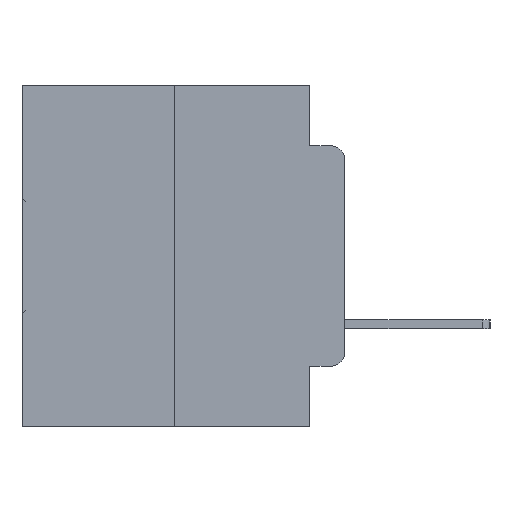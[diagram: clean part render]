
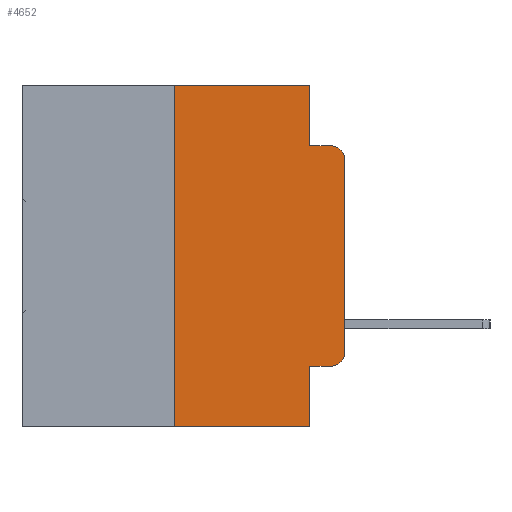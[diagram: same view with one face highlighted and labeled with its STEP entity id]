
A CAD part, left-side view. The second image highlights one B-rep face of the part: STEP entity #4652.
In plain terms, the highlighted planar face has unit normal (-1, 0, 0).
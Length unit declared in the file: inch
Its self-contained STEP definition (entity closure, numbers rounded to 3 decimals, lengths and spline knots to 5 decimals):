
#3 = ORIENTED_EDGE ( 'NONE', *, *, #9504, .F. ) ;
#164 = LINE ( 'NONE', #7670, #29394 ) ;
#460 = EDGE_CURVE ( 'NONE', #24137, #20980, #17345, .T. ) ;
#507 = VERTEX_POINT ( 'NONE', #9055 ) ;
#693 = LINE ( 'NONE', #4307, #24774 ) ;
#829 = VERTEX_POINT ( 'NONE', #10100 ) ;
#1469 = EDGE_CURVE ( 'NONE', #29351, #12513, #18439, .T. ) ;
#1563 = AXIS2_PLACEMENT_3D ( 'NONE', #19869, #17249, #2121 ) ;
#1750 = VECTOR ( 'NONE', #28447, 39.37008 ) ;
#2052 = EDGE_CURVE ( 'NONE', #29351, #24137, #27473, .T. ) ;
#2121 = DIRECTION ( 'NONE',  ( 0., 0., -1. ) ) ;
#2482 = CIRCLE ( 'NONE', #19789, 0.02 ) ;
#4156 = LINE ( 'NONE', #16186, #27305 ) ;
#4307 = CARTESIAN_POINT ( 'NONE',  ( 0., 0.051, -0.0885 ) ) ;
#4398 = LINE ( 'NONE', #22246, #21692 ) ;
#4652 = ADVANCED_FACE ( 'NONE', ( #13198 ), #22043, .F. ) ;
#4811 = ORIENTED_EDGE ( 'NONE', *, *, #11103, .F. ) ;
#5199 = CARTESIAN_POINT ( 'NONE',  ( 0., 0.02, -0.0885 ) ) ;
#5514 = DIRECTION ( 'NONE',  ( 0., 0., -1. ) ) ;
#6791 = DIRECTION ( 'NONE',  ( 0., -1., 0. ) ) ;
#6824 = DIRECTION ( 'NONE',  ( -1., 0., 0. ) ) ;
#7280 = CARTESIAN_POINT ( 'NONE',  ( 0., 0.051, 0. ) ) ;
#7670 = CARTESIAN_POINT ( 'NONE',  ( 0., 0., 0. ) ) ;
#8315 = DIRECTION ( 'NONE',  ( 0., 0., -1. ) ) ;
#8844 = CARTESIAN_POINT ( 'NONE',  ( 0., 0.051, -0.5 ) ) ;
#8852 = CARTESIAN_POINT ( 'NONE',  ( 0., 0.473, 0. ) ) ;
#8989 = ORIENTED_EDGE ( 'NONE', *, *, #18847, .F. ) ;
#8995 = CARTESIAN_POINT ( 'NONE',  ( 0., 0.02, -0.1085 ) ) ;
#9055 = CARTESIAN_POINT ( 'NONE',  ( 0., 0.051, -0.0885 ) ) ;
#9147 = VERTEX_POINT ( 'NONE', #5199 ) ;
#9278 = VECTOR ( 'NONE', #13189, 39.37008 ) ;
#9386 = DIRECTION ( 'NONE',  ( 0., 0., -1. ) ) ;
#9387 = ORIENTED_EDGE ( 'NONE', *, *, #1469, .F. ) ;
#9504 = EDGE_CURVE ( 'NONE', #16824, #829, #4156, .T. ) ;
#10100 = CARTESIAN_POINT ( 'NONE',  ( 0., 0.25, 0. ) ) ;
#11103 = EDGE_CURVE ( 'NONE', #14729, #507, #4398, .T. ) ;
#11410 = DIRECTION ( 'NONE',  ( 0., 0., -1. ) ) ;
#11564 = VECTOR ( 'NONE', #9386, 39.37008 ) ;
#11967 = ORIENTED_EDGE ( 'NONE', *, *, #14138, .F. ) ;
#12513 = VERTEX_POINT ( 'NONE', #8844 ) ;
#12517 = VECTOR ( 'NONE', #27121, 39.37008 ) ;
#13189 = DIRECTION ( 'NONE',  ( 0., -1., 0. ) ) ;
#13198 = FACE_OUTER_BOUND ( 'NONE', #27740, .T. ) ;
#14138 = EDGE_CURVE ( 'NONE', #829, #14729, #18649, .T. ) ;
#14540 = ORIENTED_EDGE ( 'NONE', *, *, #20436, .T. ) ;
#14729 = VERTEX_POINT ( 'NONE', #16574 ) ;
#15409 = AXIS2_PLACEMENT_3D ( 'NONE', #26516, #6824, #5514 ) ;
#15664 = ORIENTED_EDGE ( 'NONE', *, *, #2052, .T. ) ;
#16186 = CARTESIAN_POINT ( 'NONE',  ( 0., 0.25, 0. ) ) ;
#16574 = CARTESIAN_POINT ( 'NONE',  ( 0., 0.051, 0. ) ) ;
#16824 = VERTEX_POINT ( 'NONE', #26028 ) ;
#17043 = ORIENTED_EDGE ( 'NONE', *, *, #21936, .T. ) ;
#17128 = DIRECTION ( 'NONE',  ( 0., 0., 1. ) ) ;
#17249 = DIRECTION ( 'NONE',  ( 1., 0., 0. ) ) ;
#17345 = CIRCLE ( 'NONE', #15409, 0.02 ) ;
#18439 = LINE ( 'NONE', #7280, #11564 ) ;
#18559 = CARTESIAN_POINT ( 'NONE',  ( 0., 0., -0.3915 ) ) ;
#18649 = LINE ( 'NONE', #8852, #12517 ) ;
#18847 = EDGE_CURVE ( 'NONE', #507, #9147, #693, .T. ) ;
#19789 = AXIS2_PLACEMENT_3D ( 'NONE', #8995, #25082, #11410 ) ;
#19869 = CARTESIAN_POINT ( 'NONE',  ( 0., 0.473, 0. ) ) ;
#20436 = EDGE_CURVE ( 'NONE', #26903, #9147, #2482, .T. ) ;
#20558 = LINE ( 'NONE', #26275, #1750 ) ;
#20980 = VERTEX_POINT ( 'NONE', #18559 ) ;
#21044 = ORIENTED_EDGE ( 'NONE', *, *, #25642, .T. ) ;
#21692 = VECTOR ( 'NONE', #8315, 39.37008 ) ;
#21936 = EDGE_CURVE ( 'NONE', #20980, #26903, #164, .T. ) ;
#22043 = PLANE ( 'NONE',  #1563 ) ;
#22246 = CARTESIAN_POINT ( 'NONE',  ( 0., 0.051, 0. ) ) ;
#22605 = CARTESIAN_POINT ( 'NONE',  ( 0., 0.051, -0.4115 ) ) ;
#22703 = CARTESIAN_POINT ( 'NONE',  ( 0., 0.051, -0.4115 ) ) ;
#23135 = ORIENTED_EDGE ( 'NONE', *, *, #460, .T. ) ;
#24137 = VERTEX_POINT ( 'NONE', #29553 ) ;
#24774 = VECTOR ( 'NONE', #6791, 39.37008 ) ;
#25082 = DIRECTION ( 'NONE',  ( -1., 0., 0. ) ) ;
#25642 = EDGE_CURVE ( 'NONE', #16824, #12513, #20558, .T. ) ;
#26028 = CARTESIAN_POINT ( 'NONE',  ( 0., 0.25, -0.5 ) ) ;
#26275 = CARTESIAN_POINT ( 'NONE',  ( 0., 0.473, -0.5 ) ) ;
#26516 = CARTESIAN_POINT ( 'NONE',  ( 0., 0.02, -0.3915 ) ) ;
#26903 = VERTEX_POINT ( 'NONE', #29817 ) ;
#27121 = DIRECTION ( 'NONE',  ( 0., -1., 0. ) ) ;
#27305 = VECTOR ( 'NONE', #27443, 39.37008 ) ;
#27443 = DIRECTION ( 'NONE',  ( 0., 0., 1. ) ) ;
#27473 = LINE ( 'NONE', #22703, #9278 ) ;
#27740 = EDGE_LOOP ( 'NONE', ( #17043, #14540, #8989, #4811, #11967, #3, #21044, #9387, #15664, #23135 ) ) ;
#28447 = DIRECTION ( 'NONE',  ( 0., -1., 0. ) ) ;
#29351 = VERTEX_POINT ( 'NONE', #22605 ) ;
#29394 = VECTOR ( 'NONE', #17128, 39.37008 ) ;
#29553 = CARTESIAN_POINT ( 'NONE',  ( 0., 0.02, -0.4115 ) ) ;
#29817 = CARTESIAN_POINT ( 'NONE',  ( 0., 0., -0.1085 ) ) ;
